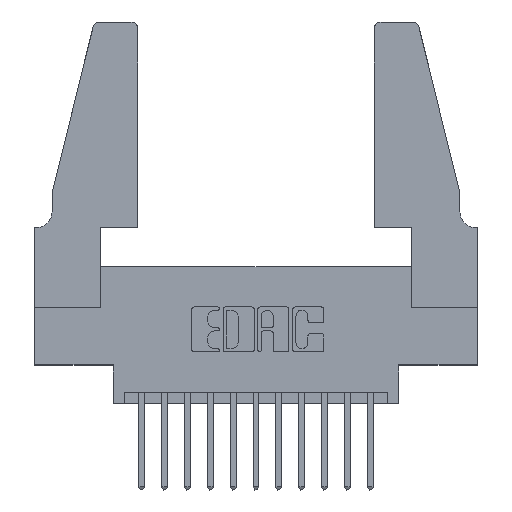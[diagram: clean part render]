
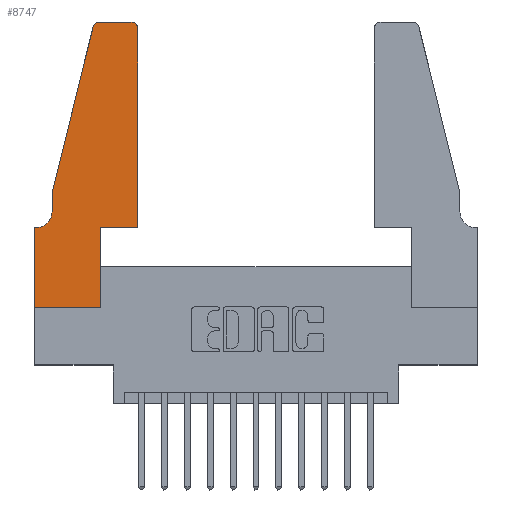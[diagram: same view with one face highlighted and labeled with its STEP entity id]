
A CAD part, top view. The second image highlights one B-rep face of the part: STEP entity #8747.
In plain terms, the highlighted planar face has unit normal (0, 0, 1).
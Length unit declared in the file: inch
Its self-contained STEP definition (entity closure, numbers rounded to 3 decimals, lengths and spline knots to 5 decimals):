
#242 = VERTEX_POINT ( 'NONE', #9613 ) ;
#255 = CARTESIAN_POINT ( 'NONE',  ( 0., 0., 0.37 ) ) ;
#480 = ORIENTED_EDGE ( 'NONE', *, *, #1323, .T. ) ;
#529 = ORIENTED_EDGE ( 'NONE', *, *, #10335, .T. ) ;
#565 = CARTESIAN_POINT ( 'NONE',  ( 0.2865, 0., 0.37 ) ) ;
#577 = FACE_OUTER_BOUND ( 'NONE', #14104, .T. ) ;
#623 = LINE ( 'NONE', #1577, #13802 ) ;
#858 = LINE ( 'NONE', #9889, #10597 ) ;
#950 = ORIENTED_EDGE ( 'NONE', *, *, #10712, .T. ) ;
#1074 = ORIENTED_EDGE ( 'NONE', *, *, #2307, .T. ) ;
#1154 = DIRECTION ( 'NONE',  ( 1., 0., 0. ) ) ;
#1323 = EDGE_CURVE ( 'NONE', #14807, #242, #3481, .T. ) ;
#1401 = CARTESIAN_POINT ( 'NONE',  ( 0.4505, 1.22, 0.37 ) ) ;
#1408 = CIRCLE ( 'NONE', #13829, 0.03 ) ;
#1577 = CARTESIAN_POINT ( 'NONE',  ( 0.4505, 0.35, 0.37 ) ) ;
#1605 = DIRECTION ( 'NONE',  ( 1., 0., 0. ) ) ;
#1794 = EDGE_CURVE ( 'NONE', #5200, #5341, #1408, .T. ) ;
#1819 = VECTOR ( 'NONE', #12834, 39.37008 ) ;
#1854 = CARTESIAN_POINT ( 'NONE',  ( 0.0755, 0.42, 0.37 ) ) ;
#1919 = VECTOR ( 'NONE', #4474, 39.37008 ) ;
#2303 = EDGE_CURVE ( 'NONE', #8352, #6746, #3261, .T. ) ;
#2307 = EDGE_CURVE ( 'NONE', #5341, #3979, #13290, .T. ) ;
#2611 = CARTESIAN_POINT ( 'NONE',  ( 0.4205, 1.22, 0.37 ) ) ;
#3191 = DIRECTION ( 'NONE',  ( 1., 0., 0. ) ) ;
#3261 = LINE ( 'NONE', #9324, #10221 ) ;
#3481 = LINE ( 'NONE', #14631, #10975 ) ;
#3621 = AXIS2_PLACEMENT_3D ( 'NONE', #11185, #11134, #9908 ) ;
#3960 = EDGE_CURVE ( 'NONE', #4978, #5200, #623, .T. ) ;
#3979 = VERTEX_POINT ( 'NONE', #13238 ) ;
#4135 = EDGE_CURVE ( 'NONE', #242, #4978, #11827, .T. ) ;
#4211 = EDGE_CURVE ( 'NONE', #9008, #12916, #11816, .T. ) ;
#4405 = DIRECTION ( 'NONE',  ( 0., 1., 0. ) ) ;
#4415 = DIRECTION ( 'NONE',  ( -0.239, -0.971, 0. ) ) ;
#4474 = DIRECTION ( 'NONE',  ( -1., 0., 0. ) ) ;
#4528 = DIRECTION ( 'NONE',  ( 0., 0., -1. ) ) ;
#4978 = VERTEX_POINT ( 'NONE', #11638 ) ;
#5200 = VERTEX_POINT ( 'NONE', #1401 ) ;
#5253 = ORIENTED_EDGE ( 'NONE', *, *, #4211, .T. ) ;
#5341 = VERTEX_POINT ( 'NONE', #11509 ) ;
#5909 = CARTESIAN_POINT ( 'NONE',  ( 0.2605, 1.25, 0.37 ) ) ;
#6746 = VERTEX_POINT ( 'NONE', #1854 ) ;
#6828 = CARTESIAN_POINT ( 'NONE',  ( 0.25487, 1.22718, 0.37 ) ) ;
#6926 = CARTESIAN_POINT ( 'NONE',  ( 0.0055, 0.42, 0.37 ) ) ;
#7068 = CIRCLE ( 'NONE', #11999, 0.07 ) ;
#7079 = DIRECTION ( 'NONE',  ( -1., 0., 0. ) ) ;
#7354 = DIRECTION ( 'NONE',  ( 0., 0., 1. ) ) ;
#7496 = ORIENTED_EDGE ( 'NONE', *, *, #11256, .T. ) ;
#7536 = DIRECTION ( 'NONE',  ( 0., 0., 1. ) ) ;
#7671 = VERTEX_POINT ( 'NONE', #255 ) ;
#7938 = CARTESIAN_POINT ( 'NONE',  ( 0.0755, 0.5, 0.37 ) ) ;
#8001 = EDGE_CURVE ( 'NONE', #7671, #14807, #13773, .T. ) ;
#8219 = CARTESIAN_POINT ( 'NONE',  ( 0., 0., 0.37 ) ) ;
#8352 = VERTEX_POINT ( 'NONE', #7938 ) ;
#8747 = ADVANCED_FACE ( 'NONE', ( #577 ), #12053, .T. ) ;
#9008 = VERTEX_POINT ( 'NONE', #11437 ) ;
#9324 = CARTESIAN_POINT ( 'NONE',  ( 0.0755, 0.5, 0.37 ) ) ;
#9613 = CARTESIAN_POINT ( 'NONE',  ( 0.2865, 0.35, 0.37 ) ) ;
#9763 = CARTESIAN_POINT ( 'NONE',  ( 0.284, 1.22, 0.37 ) ) ;
#9797 = AXIS2_PLACEMENT_3D ( 'NONE', #9763, #7536, #1605 ) ;
#9889 = CARTESIAN_POINT ( 'NONE',  ( 0.0755, 0.5, 0.37 ) ) ;
#9908 = DIRECTION ( 'NONE',  ( 1., 0., 0. ) ) ;
#10204 = CARTESIAN_POINT ( 'NONE',  ( 0.4505, 0.35, 0.37 ) ) ;
#10221 = VECTOR ( 'NONE', #13991, 39.37008 ) ;
#10273 = LINE ( 'NONE', #8219, #1819 ) ;
#10335 = EDGE_CURVE ( 'NONE', #12916, #7671, #10273, .T. ) ;
#10405 = CARTESIAN_POINT ( 'NONE',  ( 0., 0.35, 0.37 ) ) ;
#10525 = VECTOR ( 'NONE', #1154, 39.37008 ) ;
#10597 = VECTOR ( 'NONE', #4415, 39.37008 ) ;
#10615 = ORIENTED_EDGE ( 'NONE', *, *, #1794, .T. ) ;
#10712 = EDGE_CURVE ( 'NONE', #3979, #12872, #14583, .T. ) ;
#10975 = VECTOR ( 'NONE', #4405, 39.37008 ) ;
#11134 = DIRECTION ( 'NONE',  ( 0., 0., 1. ) ) ;
#11185 = CARTESIAN_POINT ( 'NONE',  ( 0., 0.35, 0.37 ) ) ;
#11212 = ORIENTED_EDGE ( 'NONE', *, *, #2303, .T. ) ;
#11256 = EDGE_CURVE ( 'NONE', #12872, #8352, #858, .T. ) ;
#11422 = CARTESIAN_POINT ( 'NONE',  ( 0.0755, 0.35, 0.37 ) ) ;
#11437 = CARTESIAN_POINT ( 'NONE',  ( 0.0055, 0.35, 0.37 ) ) ;
#11463 = ORIENTED_EDGE ( 'NONE', *, *, #13148, .T. ) ;
#11465 = VECTOR ( 'NONE', #3191, 39.37008 ) ;
#11509 = CARTESIAN_POINT ( 'NONE',  ( 0.4205, 1.25, 0.37 ) ) ;
#11638 = CARTESIAN_POINT ( 'NONE',  ( 0.4505, 0.35, 0.37 ) ) ;
#11816 = LINE ( 'NONE', #11422, #1919 ) ;
#11827 = LINE ( 'NONE', #10204, #11465 ) ;
#11999 = AXIS2_PLACEMENT_3D ( 'NONE', #6926, #4528, #13996 ) ;
#12043 = VECTOR ( 'NONE', #7079, 39.37008 ) ;
#12053 = PLANE ( 'NONE',  #3621 ) ;
#12834 = DIRECTION ( 'NONE',  ( 0., -1., 0. ) ) ;
#12872 = VERTEX_POINT ( 'NONE', #6828 ) ;
#12916 = VERTEX_POINT ( 'NONE', #10405 ) ;
#12967 = ORIENTED_EDGE ( 'NONE', *, *, #3960, .T. ) ;
#13148 = EDGE_CURVE ( 'NONE', #6746, #9008, #7068, .T. ) ;
#13238 = CARTESIAN_POINT ( 'NONE',  ( 0.284, 1.25, 0.37 ) ) ;
#13287 = DIRECTION ( 'NONE',  ( 0., 1., 0. ) ) ;
#13290 = LINE ( 'NONE', #5909, #12043 ) ;
#13773 = LINE ( 'NONE', #13982, #10525 ) ;
#13802 = VECTOR ( 'NONE', #13287, 39.37008 ) ;
#13829 = AXIS2_PLACEMENT_3D ( 'NONE', #2611, #7354, #14354 ) ;
#13982 = CARTESIAN_POINT ( 'NONE',  ( 0., 0., 0.37 ) ) ;
#13991 = DIRECTION ( 'NONE',  ( 0., -1., 0. ) ) ;
#13996 = DIRECTION ( 'NONE',  ( -1., 0., 0. ) ) ;
#14104 = EDGE_LOOP ( 'NONE', ( #1074, #950, #7496, #11212, #11463, #5253, #529, #15134, #480, #15053, #12967, #10615 ) ) ;
#14354 = DIRECTION ( 'NONE',  ( 1., 0., 0. ) ) ;
#14583 = CIRCLE ( 'NONE', #9797, 0.03 ) ;
#14631 = CARTESIAN_POINT ( 'NONE',  ( 0.2865, 0.35, 0.37 ) ) ;
#14807 = VERTEX_POINT ( 'NONE', #565 ) ;
#15053 = ORIENTED_EDGE ( 'NONE', *, *, #4135, .T. ) ;
#15134 = ORIENTED_EDGE ( 'NONE', *, *, #8001, .T. ) ;
